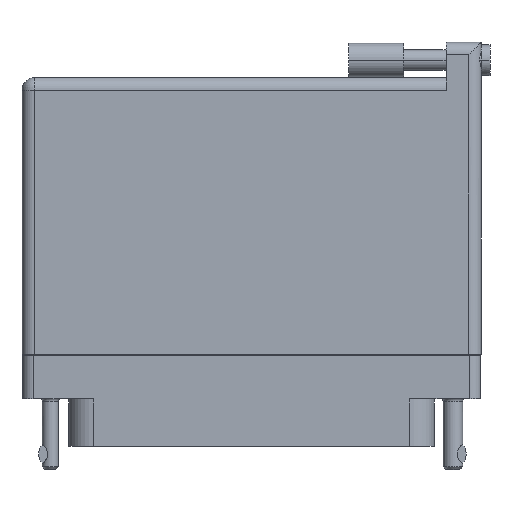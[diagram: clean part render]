
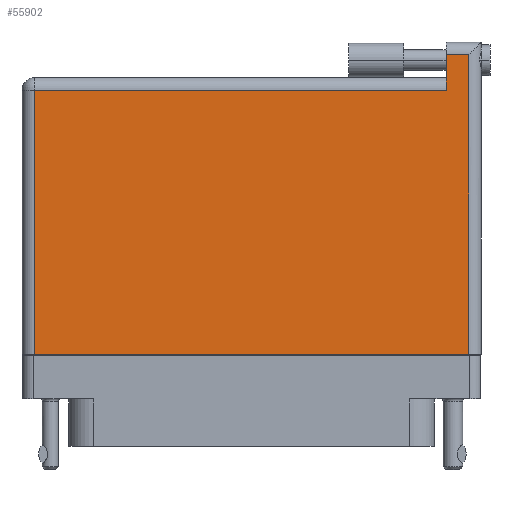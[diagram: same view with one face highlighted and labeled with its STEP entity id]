
A CAD part, front view. The second image highlights one B-rep face of the part: STEP entity #55902.
In plain terms, the highlighted face is planar.
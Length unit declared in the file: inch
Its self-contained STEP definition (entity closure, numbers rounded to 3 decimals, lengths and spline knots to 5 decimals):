
#924 = CARTESIAN_POINT ( 'NONE',  ( 1.103, 1.666, 0.4495 ) ) ;
#3526 = VECTOR ( 'NONE', #43735, 39.37008 ) ;
#4142 = VECTOR ( 'NONE', #52131, 39.37008 ) ;
#4349 = VECTOR ( 'NONE', #38575, 39.37008 ) ;
#5315 = EDGE_CURVE ( 'NONE', #40179, #56272, #26679, .T. ) ;
#6777 = EDGE_CURVE ( 'NONE', #33536, #38591, #38073, .T. ) ;
#6999 = CARTESIAN_POINT ( 'NONE',  ( -1.3, 1.396, 0.4495 ) ) ;
#7935 = CARTESIAN_POINT ( 'NONE',  ( -1.23, 1.396, 0.4495 ) ) ;
#9647 = DIRECTION ( 'NONE',  ( 0., -1., 0. ) ) ;
#10314 = EDGE_CURVE ( 'NONE', #56272, #37177, #47125, .T. ) ;
#10635 = CARTESIAN_POINT ( 'NONE',  ( 1.23, 1.596, 0.4495 ) ) ;
#11105 = EDGE_CURVE ( 'NONE', #37177, #14345, #18278, .T. ) ;
#13140 = PLANE ( 'NONE',  #42720 ) ;
#13313 = ORIENTED_EDGE ( 'NONE', *, *, #11105, .T. ) ;
#13458 = CARTESIAN_POINT ( 'NONE',  ( 1.23, 1.666, 0.4495 ) ) ;
#13729 = ORIENTED_EDGE ( 'NONE', *, *, #45804, .T. ) ;
#14345 = VERTEX_POINT ( 'NONE', #37089 ) ;
#15584 = VECTOR ( 'NONE', #37322, 39.37008 ) ;
#16051 = CARTESIAN_POINT ( 'NONE',  ( 1.23, -0.1, 0.4495 ) ) ;
#17224 = CARTESIAN_POINT ( 'NONE',  ( -1.3, 1.466, 0.4495 ) ) ;
#18278 = LINE ( 'NONE', #25701, #4142 ) ;
#19960 = VECTOR ( 'NONE', #9647, 39.37008 ) ;
#21371 = ORIENTED_EDGE ( 'NONE', *, *, #41447, .T. ) ;
#24747 = ORIENTED_EDGE ( 'NONE', *, *, #6777, .T. ) ;
#25701 = CARTESIAN_POINT ( 'NONE',  ( -1.3, 1.596, 0.4495 ) ) ;
#26679 = LINE ( 'NONE', #32855, #4349 ) ;
#27101 = VECTOR ( 'NONE', #32924, 39.37008 ) ;
#28191 = LINE ( 'NONE', #924, #19960 ) ;
#29302 = CARTESIAN_POINT ( 'NONE',  ( -1.23, -0.1, 0.4495 ) ) ;
#30814 = FACE_OUTER_BOUND ( 'NONE', #33551, .T. ) ;
#31205 = CARTESIAN_POINT ( 'NONE',  ( -1.23, -0.1, 0.4495 ) ) ;
#32855 = CARTESIAN_POINT ( 'NONE',  ( -1.3, -0.1, 0.4495 ) ) ;
#32924 = DIRECTION ( 'NONE',  ( 0., -1., 0. ) ) ;
#33536 = VERTEX_POINT ( 'NONE', #47862 ) ;
#33551 = EDGE_LOOP ( 'NONE', ( #50007, #51979, #13313, #21371, #24747, #13729 ) ) ;
#34540 = DIRECTION ( 'NONE',  ( -1., 0., 0. ) ) ;
#34912 = DIRECTION ( 'NONE',  ( 0., 0., -1. ) ) ;
#37089 = CARTESIAN_POINT ( 'NONE',  ( 1.103, 1.596, 0.4495 ) ) ;
#37177 = VERTEX_POINT ( 'NONE', #10635 ) ;
#37322 = DIRECTION ( 'NONE',  ( -1., 0., 0. ) ) ;
#38073 = LINE ( 'NONE', #6999, #15584 ) ;
#38575 = DIRECTION ( 'NONE',  ( 1., 0., 0. ) ) ;
#38591 = VERTEX_POINT ( 'NONE', #7935 ) ;
#40179 = VERTEX_POINT ( 'NONE', #29302 ) ;
#41447 = EDGE_CURVE ( 'NONE', #14345, #33536, #28191, .T. ) ;
#42720 = AXIS2_PLACEMENT_3D ( 'NONE', #17224, #34912, #34540 ) ;
#43735 = DIRECTION ( 'NONE',  ( 0., 1., 0. ) ) ;
#45804 = EDGE_CURVE ( 'NONE', #38591, #40179, #50385, .T. ) ;
#47125 = LINE ( 'NONE', #13458, #3526 ) ;
#47862 = CARTESIAN_POINT ( 'NONE',  ( 1.103, 1.396, 0.4495 ) ) ;
#50007 = ORIENTED_EDGE ( 'NONE', *, *, #5315, .T. ) ;
#50385 = LINE ( 'NONE', #31205, #27101 ) ;
#51979 = ORIENTED_EDGE ( 'NONE', *, *, #10314, .T. ) ;
#52131 = DIRECTION ( 'NONE',  ( -1., 0., 0. ) ) ;
#55902 = ADVANCED_FACE ( 'NONE', ( #30814 ), #13140, .F. ) ;
#56272 = VERTEX_POINT ( 'NONE', #16051 ) ;
